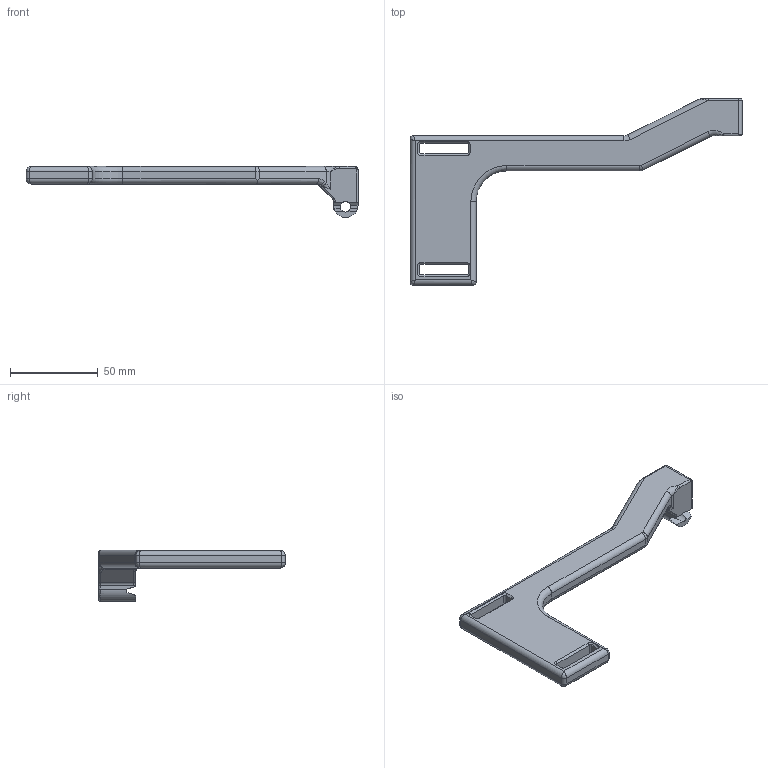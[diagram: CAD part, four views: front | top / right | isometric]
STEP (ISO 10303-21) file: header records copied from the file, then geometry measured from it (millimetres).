
FILE_DESCRIPTION(/* description */ (''),/* implementation_level */ '2;1');
FILE_NAME(/* name */ 'USW Brace.step',/* time_stamp */ '2023-02-14T18:50:36-07:00',/* author */ (''),/* organization */ (''),/* preprocessor_version */ 'ST-DEVELOPER v19.2',/* originating_system */ 'Autodesk Translation Framework v11.17.0.187',/* authorisation */ '');
FILE_SCHEMA (('AUTOMOTIVE_DESIGN { 1 0 10303 214 3 1 1 }'));
Length unit declared in the file: millimetre
Products named in the file (1): G19X
Bounding box: 188.68 x 106.03 x 29.04 mm (x, y, z)
Volume: 64478.6 mm3; surface area: 19115 mm2
Topology: 1 solids, 1 shells, 138 faces, 331 edges, 184 vertices
Faces by surface type: cylinder 47, plane 45, bspline 17, cone 17, torus 12
Full cylindrical faces by diameter (mm): 6 x1, 9 x1
Entity records: 4420 total; most frequent: CARTESIAN_POINT 1199, DIRECTION 688, ORIENTED_EDGE 642, EDGE_CURVE 321, AXIS2_PLACEMENT_3D 262, VERTEX_POINT 184, LINE 164, VECTOR 164
